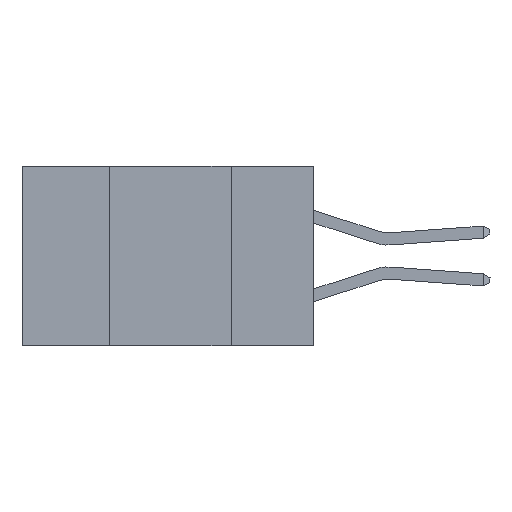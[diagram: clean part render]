
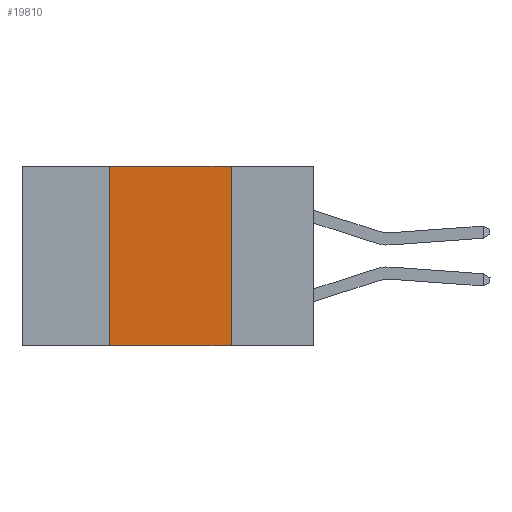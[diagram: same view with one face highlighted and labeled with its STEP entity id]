
A CAD part, left-side view. The second image highlights one B-rep face of the part: STEP entity #19810.
In plain terms, the highlighted planar face has unit normal (-1, 0, 0).
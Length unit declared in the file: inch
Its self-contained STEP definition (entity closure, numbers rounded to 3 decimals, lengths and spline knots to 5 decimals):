
#50 = ORIENTED_EDGE ( 'NONE', *, *, #32063, .F. ) ;
#359 = EDGE_LOOP ( 'NONE', ( #948, #50, #20945, #17116 ) ) ;
#628 = VECTOR ( 'NONE', #13627, 39.37008 ) ;
#948 = ORIENTED_EDGE ( 'NONE', *, *, #22197, .F. ) ;
#1226 = CARTESIAN_POINT ( 'NONE',  ( 0., 0.42, 0. ) ) ;
#5681 = EDGE_CURVE ( 'NONE', #9149, #10077, #33803, .T. ) ;
#6441 = DIRECTION ( 'NONE',  ( 0., 0., 1. ) ) ;
#9149 = VERTEX_POINT ( 'NONE', #28322 ) ;
#9340 = AXIS2_PLACEMENT_3D ( 'NONE', #25317, #15569, #9553 ) ;
#9553 = DIRECTION ( 'NONE',  ( 0., 0., -1. ) ) ;
#10077 = VERTEX_POINT ( 'NONE', #20584 ) ;
#11137 = CARTESIAN_POINT ( 'NONE',  ( 0., 0.6, 0. ) ) ;
#13627 = DIRECTION ( 'NONE',  ( 0., 0., -1. ) ) ;
#14427 = VECTOR ( 'NONE', #6441, 39.37008 ) ;
#15569 = DIRECTION ( 'NONE',  ( 1., 0., 0. ) ) ;
#17116 = ORIENTED_EDGE ( 'NONE', *, *, #23145, .T. ) ;
#17812 = VERTEX_POINT ( 'NONE', #22654 ) ;
#18765 = CARTESIAN_POINT ( 'NONE',  ( 0., 0.17, 0. ) ) ;
#19810 = ADVANCED_FACE ( 'NONE', ( #20785 ), #22672, .F. ) ;
#20584 = CARTESIAN_POINT ( 'NONE',  ( 0., 0.42, 0. ) ) ;
#20785 = FACE_OUTER_BOUND ( 'NONE', #359, .T. ) ;
#20945 = ORIENTED_EDGE ( 'NONE', *, *, #5681, .F. ) ;
#21572 = DIRECTION ( 'NONE',  ( 0., -1., 0. ) ) ;
#22197 = EDGE_CURVE ( 'NONE', #24933, #17812, #28829, .T. ) ;
#22654 = CARTESIAN_POINT ( 'NONE',  ( 0., 0.17, -0.37 ) ) ;
#22672 = PLANE ( 'NONE',  #9340 ) ;
#23145 = EDGE_CURVE ( 'NONE', #9149, #17812, #33333, .T. ) ;
#24933 = VERTEX_POINT ( 'NONE', #25810 ) ;
#25317 = CARTESIAN_POINT ( 'NONE',  ( 0., 0.6, 0. ) ) ;
#25810 = CARTESIAN_POINT ( 'NONE',  ( 0., 0.17, 0. ) ) ;
#25845 = CARTESIAN_POINT ( 'NONE',  ( 0., 0.6, -0.37 ) ) ;
#25958 = DIRECTION ( 'NONE',  ( 0., -1., 0. ) ) ;
#28322 = CARTESIAN_POINT ( 'NONE',  ( 0., 0.42, -0.37 ) ) ;
#28829 = LINE ( 'NONE', #18765, #628 ) ;
#29706 = VECTOR ( 'NONE', #21572, 39.37008 ) ;
#31286 = VECTOR ( 'NONE', #25958, 39.37008 ) ;
#32063 = EDGE_CURVE ( 'NONE', #10077, #24933, #32629, .T. ) ;
#32629 = LINE ( 'NONE', #11137, #29706 ) ;
#33333 = LINE ( 'NONE', #25845, #31286 ) ;
#33803 = LINE ( 'NONE', #1226, #14427 ) ;
